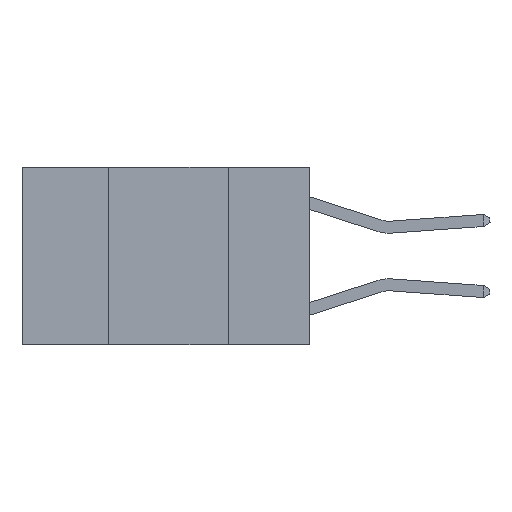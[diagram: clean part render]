
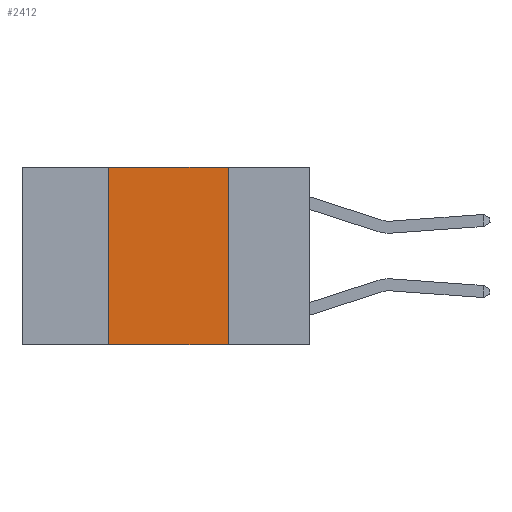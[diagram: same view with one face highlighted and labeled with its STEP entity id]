
A CAD part, left-side view. The second image highlights one B-rep face of the part: STEP entity #2412.
In plain terms, the highlighted planar face has unit normal (-1, 0, 0).
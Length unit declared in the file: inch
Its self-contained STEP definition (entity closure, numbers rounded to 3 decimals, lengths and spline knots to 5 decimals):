
#8 = CARTESIAN_POINT ( 'NONE',  ( 0., 0.6, 0. ) ) ;
#130 = CARTESIAN_POINT ( 'NONE',  ( 0., 0.42, -0.37 ) ) ;
#226 = ORIENTED_EDGE ( 'NONE', *, *, #3834, .T. ) ;
#388 = VERTEX_POINT ( 'NONE', #2434 ) ;
#433 = LINE ( 'NONE', #2986, #10083 ) ;
#1128 = AXIS2_PLACEMENT_3D ( 'NONE', #8, #3511, #9457 ) ;
#1210 = ORIENTED_EDGE ( 'NONE', *, *, #10835, .F. ) ;
#1876 = DIRECTION ( 'NONE',  ( 0., -1., 0. ) ) ;
#2293 = LINE ( 'NONE', #3589, #6907 ) ;
#2412 = ADVANCED_FACE ( 'NONE', ( #7464 ), #8611, .F. ) ;
#2434 = CARTESIAN_POINT ( 'NONE',  ( 0., 0.42, 0. ) ) ;
#2650 = EDGE_CURVE ( 'NONE', #7494, #388, #433, .T. ) ;
#2782 = LINE ( 'NONE', #9843, #5120 ) ;
#2986 = CARTESIAN_POINT ( 'NONE',  ( 0., 0.42, 0. ) ) ;
#3511 = DIRECTION ( 'NONE',  ( 1., 0., 0. ) ) ;
#3581 = CARTESIAN_POINT ( 'NONE',  ( 0., 0.17, 0. ) ) ;
#3589 = CARTESIAN_POINT ( 'NONE',  ( 0., 0.6, -0.37 ) ) ;
#3834 = EDGE_CURVE ( 'NONE', #7494, #10649, #2293, .T. ) ;
#3909 = DIRECTION ( 'NONE',  ( 0., -1., 0. ) ) ;
#4666 = DIRECTION ( 'NONE',  ( 0., 0., -1. ) ) ;
#4883 = LINE ( 'NONE', #6386, #7163 ) ;
#5067 = EDGE_LOOP ( 'NONE', ( #1210, #9739, #8423, #226 ) ) ;
#5120 = VECTOR ( 'NONE', #3909, 39.37008 ) ;
#6386 = CARTESIAN_POINT ( 'NONE',  ( 0., 0.17, 0. ) ) ;
#6522 = EDGE_CURVE ( 'NONE', #388, #10046, #2782, .T. ) ;
#6907 = VECTOR ( 'NONE', #1876, 39.37008 ) ;
#7163 = VECTOR ( 'NONE', #4666, 39.37008 ) ;
#7464 = FACE_OUTER_BOUND ( 'NONE', #5067, .T. ) ;
#7494 = VERTEX_POINT ( 'NONE', #130 ) ;
#8423 = ORIENTED_EDGE ( 'NONE', *, *, #2650, .F. ) ;
#8611 = PLANE ( 'NONE',  #1128 ) ;
#8979 = DIRECTION ( 'NONE',  ( 0., 0., 1. ) ) ;
#9457 = DIRECTION ( 'NONE',  ( 0., 0., -1. ) ) ;
#9515 = CARTESIAN_POINT ( 'NONE',  ( 0., 0.17, -0.37 ) ) ;
#9739 = ORIENTED_EDGE ( 'NONE', *, *, #6522, .F. ) ;
#9843 = CARTESIAN_POINT ( 'NONE',  ( 0., 0.6, 0. ) ) ;
#10046 = VERTEX_POINT ( 'NONE', #3581 ) ;
#10083 = VECTOR ( 'NONE', #8979, 39.37008 ) ;
#10649 = VERTEX_POINT ( 'NONE', #9515 ) ;
#10835 = EDGE_CURVE ( 'NONE', #10046, #10649, #4883, .T. ) ;
